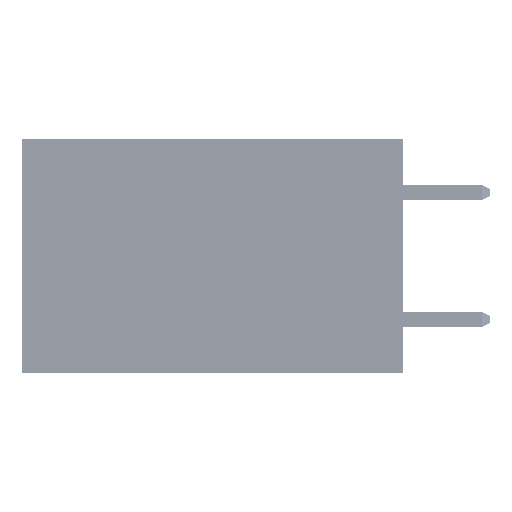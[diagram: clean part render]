
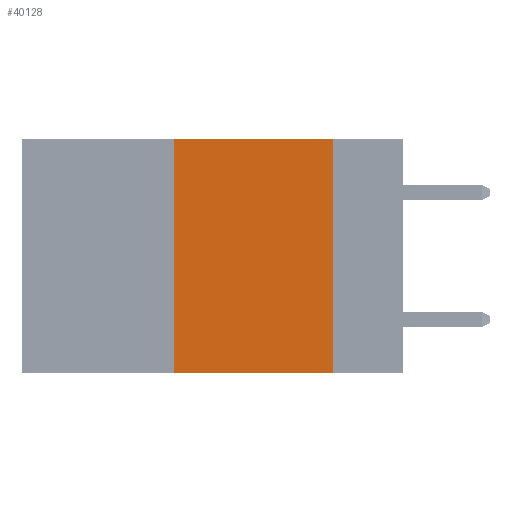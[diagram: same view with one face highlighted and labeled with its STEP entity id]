
A CAD part, left-side view. The second image highlights one B-rep face of the part: STEP entity #40128.
In plain terms, the highlighted planar face has unit normal (-1, 0, 0).
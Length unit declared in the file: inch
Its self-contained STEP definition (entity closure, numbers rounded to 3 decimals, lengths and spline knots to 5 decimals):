
#254 = VERTEX_POINT ( 'NONE', #34308 ) ;
#1493 = ORIENTED_EDGE ( 'NONE', *, *, #16006, .F. ) ;
#1817 = DIRECTION ( 'NONE',  ( 0., 0., -1. ) ) ;
#4525 = AXIS2_PLACEMENT_3D ( 'NONE', #13740, #26041, #1817 ) ;
#4991 = LINE ( 'NONE', #30326, #17750 ) ;
#5923 = DIRECTION ( 'NONE',  ( 0., -1., 0. ) ) ;
#7575 = EDGE_CURVE ( 'NONE', #19359, #51056, #29081, .T. ) ;
#7590 = CARTESIAN_POINT ( 'NONE',  ( 0., 0.11, 0. ) ) ;
#10452 = CARTESIAN_POINT ( 'NONE',  ( 0., 0.11, -0.37 ) ) ;
#11638 = EDGE_CURVE ( 'NONE', #254, #26952, #4991, .T. ) ;
#11740 = ORIENTED_EDGE ( 'NONE', *, *, #11638, .F. ) ;
#13740 = CARTESIAN_POINT ( 'NONE',  ( 0., 0.6, 0. ) ) ;
#16006 = EDGE_CURVE ( 'NONE', #19359, #254, #35600, .T. ) ;
#17750 = VECTOR ( 'NONE', #5923, 39.37008 ) ;
#18982 = CARTESIAN_POINT ( 'NONE',  ( 0., 0.11, 0. ) ) ;
#19359 = VERTEX_POINT ( 'NONE', #32710 ) ;
#20073 = DIRECTION ( 'NONE',  ( 0., -1., 0. ) ) ;
#24914 = VECTOR ( 'NONE', #34781, 39.37008 ) ;
#26041 = DIRECTION ( 'NONE',  ( 1., 0., 0. ) ) ;
#26804 = LINE ( 'NONE', #18982, #24914 ) ;
#26952 = VERTEX_POINT ( 'NONE', #7590 ) ;
#29081 = LINE ( 'NONE', #36570, #32264 ) ;
#29405 = CARTESIAN_POINT ( 'NONE',  ( 0., 0.36, 0. ) ) ;
#30326 = CARTESIAN_POINT ( 'NONE',  ( 0., 0.6, 0. ) ) ;
#32264 = VECTOR ( 'NONE', #20073, 39.37008 ) ;
#32366 = EDGE_CURVE ( 'NONE', #26952, #51056, #26804, .T. ) ;
#32710 = CARTESIAN_POINT ( 'NONE',  ( 0., 0.36, -0.37 ) ) ;
#32932 = ORIENTED_EDGE ( 'NONE', *, *, #32366, .F. ) ;
#34308 = CARTESIAN_POINT ( 'NONE',  ( 0., 0.36, 0. ) ) ;
#34781 = DIRECTION ( 'NONE',  ( 0., 0., -1. ) ) ;
#35600 = LINE ( 'NONE', #29405, #45135 ) ;
#36570 = CARTESIAN_POINT ( 'NONE',  ( 0., 0.6, -0.37 ) ) ;
#40128 = ADVANCED_FACE ( 'NONE', ( #49740 ), #46627, .F. ) ;
#45135 = VECTOR ( 'NONE', #50289, 39.37008 ) ;
#46627 = PLANE ( 'NONE',  #4525 ) ;
#49740 = FACE_OUTER_BOUND ( 'NONE', #50003, .T. ) ;
#50003 = EDGE_LOOP ( 'NONE', ( #32932, #11740, #1493, #50715 ) ) ;
#50289 = DIRECTION ( 'NONE',  ( 0., 0., 1. ) ) ;
#50715 = ORIENTED_EDGE ( 'NONE', *, *, #7575, .T. ) ;
#51056 = VERTEX_POINT ( 'NONE', #10452 ) ;
